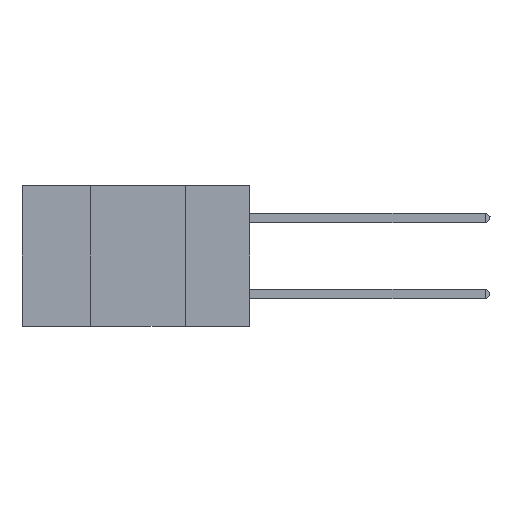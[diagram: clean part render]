
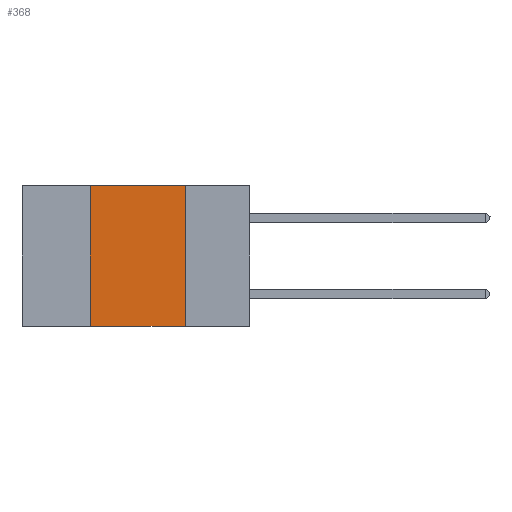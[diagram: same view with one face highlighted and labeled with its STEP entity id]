
A CAD part, left-side view. The second image highlights one B-rep face of the part: STEP entity #368.
In plain terms, the highlighted planar face has unit normal (-1, 0, 0).
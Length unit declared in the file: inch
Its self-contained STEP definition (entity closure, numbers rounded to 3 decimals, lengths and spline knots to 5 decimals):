
#317 = CARTESIAN_POINT ( 'NONE',  ( 0., 0.42, -0.37 ) ) ;
#368 = ADVANCED_FACE ( 'NONE', ( #5587 ), #2496, .F. ) ;
#376 = CARTESIAN_POINT ( 'NONE',  ( 0., 0.17, -0.37 ) ) ;
#901 = ORIENTED_EDGE ( 'NONE', *, *, #12433, .T. ) ;
#1028 = CARTESIAN_POINT ( 'NONE',  ( 0., 0.42, 0. ) ) ;
#1260 = LINE ( 'NONE', #11699, #8684 ) ;
#1602 = VERTEX_POINT ( 'NONE', #12325 ) ;
#1654 = EDGE_LOOP ( 'NONE', ( #2546, #2790, #7469, #901 ) ) ;
#2020 = DIRECTION ( 'NONE',  ( 0., -1., 0. ) ) ;
#2496 = PLANE ( 'NONE',  #8188 ) ;
#2546 = ORIENTED_EDGE ( 'NONE', *, *, #6617, .F. ) ;
#2790 = ORIENTED_EDGE ( 'NONE', *, *, #11176, .F. ) ;
#2870 = EDGE_CURVE ( 'NONE', #10914, #9669, #10712, .T. ) ;
#3204 = DIRECTION ( 'NONE',  ( 0., -1., 0. ) ) ;
#3461 = DIRECTION ( 'NONE',  ( 0., 0., 1. ) ) ;
#4465 = CARTESIAN_POINT ( 'NONE',  ( 0., 0.42, 0. ) ) ;
#4496 = CARTESIAN_POINT ( 'NONE',  ( 0., 0.6, 0. ) ) ;
#4570 = DIRECTION ( 'NONE',  ( 0., 0., -1. ) ) ;
#5428 = LINE ( 'NONE', #9305, #8500 ) ;
#5587 = FACE_OUTER_BOUND ( 'NONE', #1654, .T. ) ;
#6596 = DIRECTION ( 'NONE',  ( 1., 0., 0. ) ) ;
#6617 = EDGE_CURVE ( 'NONE', #1602, #9454, #1260, .T. ) ;
#6643 = DIRECTION ( 'NONE',  ( 0., 0., -1. ) ) ;
#7309 = CARTESIAN_POINT ( 'NONE',  ( 0., 0.6, 0. ) ) ;
#7469 = ORIENTED_EDGE ( 'NONE', *, *, #2870, .F. ) ;
#8188 = AXIS2_PLACEMENT_3D ( 'NONE', #4496, #6596, #4570 ) ;
#8500 = VECTOR ( 'NONE', #3204, 39.37008 ) ;
#8684 = VECTOR ( 'NONE', #6643, 39.37008 ) ;
#8689 = VECTOR ( 'NONE', #3461, 39.37008 ) ;
#9305 = CARTESIAN_POINT ( 'NONE',  ( 0., 0.6, -0.37 ) ) ;
#9454 = VERTEX_POINT ( 'NONE', #376 ) ;
#9669 = VERTEX_POINT ( 'NONE', #1028 ) ;
#10712 = LINE ( 'NONE', #4465, #8689 ) ;
#10914 = VERTEX_POINT ( 'NONE', #317 ) ;
#11176 = EDGE_CURVE ( 'NONE', #9669, #1602, #11358, .T. ) ;
#11358 = LINE ( 'NONE', #7309, #13049 ) ;
#11699 = CARTESIAN_POINT ( 'NONE',  ( 0., 0.17, 0. ) ) ;
#12325 = CARTESIAN_POINT ( 'NONE',  ( 0., 0.17, 0. ) ) ;
#12433 = EDGE_CURVE ( 'NONE', #10914, #9454, #5428, .T. ) ;
#13049 = VECTOR ( 'NONE', #2020, 39.37008 ) ;
